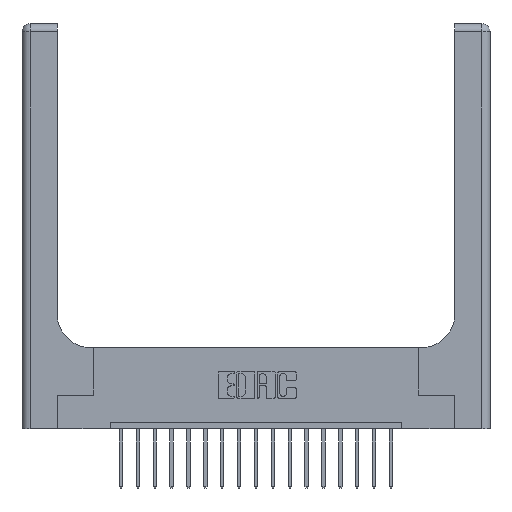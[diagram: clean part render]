
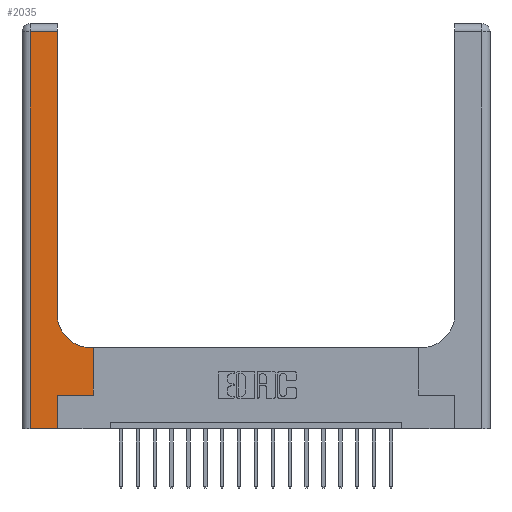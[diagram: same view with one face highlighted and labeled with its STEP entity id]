
A CAD part, top view. The second image highlights one B-rep face of the part: STEP entity #2035.
In plain terms, the highlighted planar face has unit normal (0, 0, 1).
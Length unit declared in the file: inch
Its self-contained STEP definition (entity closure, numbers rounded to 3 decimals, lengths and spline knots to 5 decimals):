
#40 = EDGE_CURVE ( 'NONE', #14216, #4448, #15524, .T. ) ;
#374 = LINE ( 'NONE', #5513, #15605 ) ;
#473 = LINE ( 'NONE', #10490, #4875 ) ;
#565 = AXIS2_PLACEMENT_3D ( 'NONE', #6444, #10902, #10839 ) ;
#694 = ORIENTED_EDGE ( 'NONE', *, *, #1783, .T. ) ;
#797 = VERTEX_POINT ( 'NONE', #16215 ) ;
#802 = DIRECTION ( 'NONE',  ( 0., 1., 0. ) ) ;
#1036 = ORIENTED_EDGE ( 'NONE', *, *, #40, .T. ) ;
#1403 = AXIS2_PLACEMENT_3D ( 'NONE', #10128, #17672, #8821 ) ;
#1643 = CARTESIAN_POINT ( 'NONE',  ( 0.06, 3., 0.37 ) ) ;
#1783 = EDGE_CURVE ( 'NONE', #10645, #10610, #12482, .T. ) ;
#1851 = CARTESIAN_POINT ( 'NONE',  ( 0., 0., 0.37 ) ) ;
#2035 = ADVANCED_FACE ( 'NONE', ( #14762 ), #7342, .F. ) ;
#2148 = CARTESIAN_POINT ( 'NONE',  ( 0.06, 2.94, 0.37 ) ) ;
#2692 = VECTOR ( 'NONE', #16964, 39.37008 ) ;
#2824 = VERTEX_POINT ( 'NONE', #2148 ) ;
#3121 = CARTESIAN_POINT ( 'NONE',  ( 0.26, 0.85, 0.37 ) ) ;
#3424 = EDGE_LOOP ( 'NONE', ( #13750, #18997, #7217, #694, #14585, #1036, #11187, #12049, #15643 ) ) ;
#3542 = LINE ( 'NONE', #16092, #5633 ) ;
#4370 = DIRECTION ( 'NONE',  ( -1., 0., 0. ) ) ;
#4448 = VERTEX_POINT ( 'NONE', #17460 ) ;
#4576 = EDGE_CURVE ( 'NONE', #8303, #10227, #13299, .T. ) ;
#4875 = VECTOR ( 'NONE', #8997, 39.37008 ) ;
#5222 = CARTESIAN_POINT ( 'NONE',  ( 0.51, 0.6, 0.37 ) ) ;
#5513 = CARTESIAN_POINT ( 'NONE',  ( 0.26, 3., 0.37 ) ) ;
#5633 = VECTOR ( 'NONE', #4370, 39.37008 ) ;
#6310 = CARTESIAN_POINT ( 'NONE',  ( 0.265, 0.25, 0.37 ) ) ;
#6444 = CARTESIAN_POINT ( 'NONE',  ( 0.51, 0.85, 0.37 ) ) ;
#6693 = CARTESIAN_POINT ( 'NONE',  ( 0.265, 0.25, 0.37 ) ) ;
#7217 = ORIENTED_EDGE ( 'NONE', *, *, #14341, .T. ) ;
#7342 = PLANE ( 'NONE',  #1403 ) ;
#7397 = VECTOR ( 'NONE', #16753, 39.37008 ) ;
#7452 = LINE ( 'NONE', #1643, #8837 ) ;
#7599 = EDGE_CURVE ( 'NONE', #797, #8303, #11034, .T. ) ;
#7709 = EDGE_CURVE ( 'NONE', #10227, #13626, #374, .T. ) ;
#7770 = DIRECTION ( 'NONE',  ( 0., 1., 0. ) ) ;
#8303 = VERTEX_POINT ( 'NONE', #5222 ) ;
#8590 = CARTESIAN_POINT ( 'NONE',  ( 0.265, 0., 0.37 ) ) ;
#8821 = DIRECTION ( 'NONE',  ( -1., 0., 0. ) ) ;
#8837 = VECTOR ( 'NONE', #11870, 39.37008 ) ;
#8839 = LINE ( 'NONE', #11437, #16441 ) ;
#8997 = DIRECTION ( 'NONE',  ( 0., 1., 0. ) ) ;
#9484 = DIRECTION ( 'NONE',  ( 1., 0., 0. ) ) ;
#9667 = EDGE_CURVE ( 'NONE', #10610, #14216, #8839, .T. ) ;
#9751 = CARTESIAN_POINT ( 'NONE',  ( 0.06, 0., 0.37 ) ) ;
#10128 = CARTESIAN_POINT ( 'NONE',  ( 0., 3., 0.37 ) ) ;
#10227 = VERTEX_POINT ( 'NONE', #3121 ) ;
#10490 = CARTESIAN_POINT ( 'NONE',  ( 0.528, 0.25, 0.37 ) ) ;
#10610 = VERTEX_POINT ( 'NONE', #8590 ) ;
#10645 = VERTEX_POINT ( 'NONE', #9751 ) ;
#10839 = DIRECTION ( 'NONE',  ( 1., 0., 0. ) ) ;
#10902 = DIRECTION ( 'NONE',  ( 0., 0., -1. ) ) ;
#11034 = LINE ( 'NONE', #16708, #2692 ) ;
#11187 = ORIENTED_EDGE ( 'NONE', *, *, #16021, .T. ) ;
#11437 = CARTESIAN_POINT ( 'NONE',  ( 0.265, 0., 0.37 ) ) ;
#11634 = VECTOR ( 'NONE', #9484, 39.37008 ) ;
#11870 = DIRECTION ( 'NONE',  ( 0., -1., 0. ) ) ;
#12049 = ORIENTED_EDGE ( 'NONE', *, *, #7599, .T. ) ;
#12482 = LINE ( 'NONE', #1851, #7397 ) ;
#13299 = CIRCLE ( 'NONE', #565, 0.25 ) ;
#13481 = EDGE_CURVE ( 'NONE', #13626, #2824, #3542, .T. ) ;
#13626 = VERTEX_POINT ( 'NONE', #13786 ) ;
#13750 = ORIENTED_EDGE ( 'NONE', *, *, #7709, .T. ) ;
#13786 = CARTESIAN_POINT ( 'NONE',  ( 0.26, 2.94, 0.37 ) ) ;
#14216 = VERTEX_POINT ( 'NONE', #6693 ) ;
#14341 = EDGE_CURVE ( 'NONE', #2824, #10645, #7452, .T. ) ;
#14585 = ORIENTED_EDGE ( 'NONE', *, *, #9667, .T. ) ;
#14762 = FACE_OUTER_BOUND ( 'NONE', #3424, .T. ) ;
#15524 = LINE ( 'NONE', #6310, #11634 ) ;
#15605 = VECTOR ( 'NONE', #802, 39.37008 ) ;
#15643 = ORIENTED_EDGE ( 'NONE', *, *, #4576, .T. ) ;
#16021 = EDGE_CURVE ( 'NONE', #4448, #797, #473, .T. ) ;
#16092 = CARTESIAN_POINT ( 'NONE',  ( 0., 2.94, 0.37 ) ) ;
#16215 = CARTESIAN_POINT ( 'NONE',  ( 0.528, 0.6, 0.37 ) ) ;
#16441 = VECTOR ( 'NONE', #7770, 39.37008 ) ;
#16708 = CARTESIAN_POINT ( 'NONE',  ( 0.26, 0.6, 0.37 ) ) ;
#16753 = DIRECTION ( 'NONE',  ( 1., 0., 0. ) ) ;
#16964 = DIRECTION ( 'NONE',  ( -1., 0., 0. ) ) ;
#17460 = CARTESIAN_POINT ( 'NONE',  ( 0.528, 0.25, 0.37 ) ) ;
#17672 = DIRECTION ( 'NONE',  ( 0., 0., -1. ) ) ;
#18997 = ORIENTED_EDGE ( 'NONE', *, *, #13481, .T. ) ;
